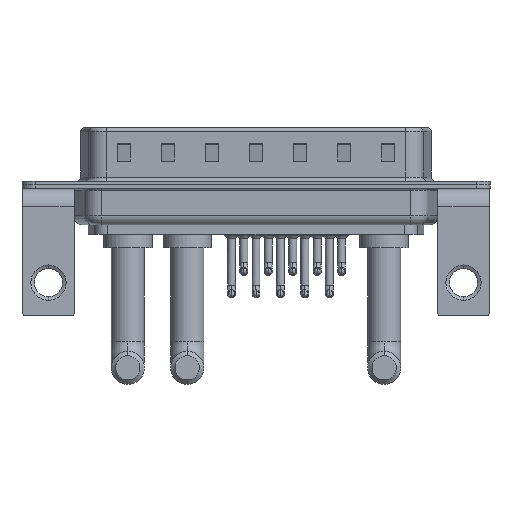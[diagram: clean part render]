
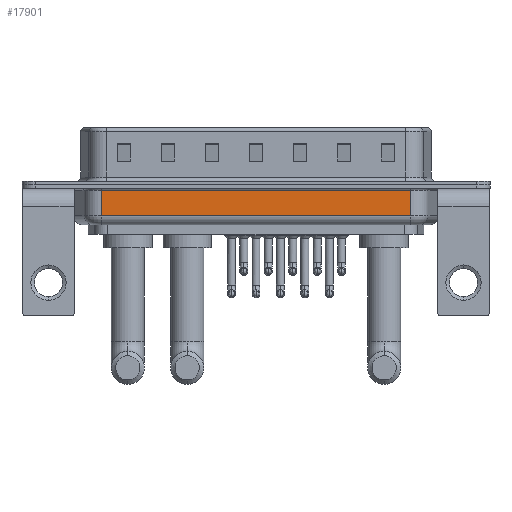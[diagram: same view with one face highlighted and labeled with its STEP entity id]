
A CAD part, front view. The second image highlights one B-rep face of the part: STEP entity #17901.
In plain terms, the highlighted planar face has unit normal (0, -1, 0).
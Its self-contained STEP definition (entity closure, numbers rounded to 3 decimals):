
#72 = VERTEX_POINT ( 'NONE', #9048 ) ;
#612 = CARTESIAN_POINT ( 'NONE',  ( 41.044, -5.35, -4.5 ) ) ;
#1063 = EDGE_CURVE ( 'NONE', #22351, #6361, #1485, .T. ) ;
#1106 = DIRECTION ( 'NONE',  ( 0., 0., 1. ) ) ;
#1122 = VECTOR ( 'NONE', #11524, 1000. ) ;
#1485 = LINE ( 'NONE', #7464, #18608 ) ;
#2270 = EDGE_CURVE ( 'NONE', #22351, #7087, #5910, .T. ) ;
#3722 = DIRECTION ( 'NONE',  ( 0., 0., 1. ) ) ;
#4683 = ORIENTED_EDGE ( 'NONE', *, *, #1063, .F. ) ;
#5135 = VECTOR ( 'NONE', #9587, 1000. ) ;
#5910 = LINE ( 'NONE', #15371, #7220 ) ;
#6139 = ORIENTED_EDGE ( 'NONE', *, *, #2270, .T. ) ;
#6293 = ORIENTED_EDGE ( 'NONE', *, *, #15575, .T. ) ;
#6361 = VERTEX_POINT ( 'NONE', #6918 ) ;
#6918 = CARTESIAN_POINT ( 'NONE',  ( 6.006, -5.35, -0.65 ) ) ;
#7087 = VERTEX_POINT ( 'NONE', #23111 ) ;
#7220 = VECTOR ( 'NONE', #13510, 1000. ) ;
#7464 = CARTESIAN_POINT ( 'NONE',  ( 6.006, -5.35, -4.5 ) ) ;
#9048 = CARTESIAN_POINT ( 'NONE',  ( 41.044, -5.35, -0.65 ) ) ;
#9587 = DIRECTION ( 'NONE',  ( 0., 0., 1. ) ) ;
#11524 = DIRECTION ( 'NONE',  ( -1., 0., 0. ) ) ;
#12431 = EDGE_LOOP ( 'NONE', ( #4683, #6139, #12727, #6293 ) ) ;
#12727 = ORIENTED_EDGE ( 'NONE', *, *, #16461, .T. ) ;
#13343 = LINE ( 'NONE', #612, #5135 ) ;
#13510 = DIRECTION ( 'NONE',  ( 1., 0., 0. ) ) ;
#14078 = CARTESIAN_POINT ( 'NONE',  ( 6.006, -5.35, -4.5 ) ) ;
#15163 = LINE ( 'NONE', #20838, #1122 ) ;
#15371 = CARTESIAN_POINT ( 'NONE',  ( 6.006, -5.35, -3.5 ) ) ;
#15575 = EDGE_CURVE ( 'NONE', #72, #6361, #15163, .T. ) ;
#15919 = PLANE ( 'NONE',  #16711 ) ;
#16461 = EDGE_CURVE ( 'NONE', #7087, #72, #13343, .T. ) ;
#16711 = AXIS2_PLACEMENT_3D ( 'NONE', #14078, #18139, #1106 ) ;
#17901 = ADVANCED_FACE ( 'NONE', ( #23459 ), #15919, .F. ) ;
#18139 = DIRECTION ( 'NONE',  ( 0., 1., 0. ) ) ;
#18608 = VECTOR ( 'NONE', #3722, 1000. ) ;
#18840 = CARTESIAN_POINT ( 'NONE',  ( 6.006, -5.35, -3.5 ) ) ;
#20838 = CARTESIAN_POINT ( 'NONE',  ( 6.006, -5.35, -0.65 ) ) ;
#22351 = VERTEX_POINT ( 'NONE', #18840 ) ;
#23111 = CARTESIAN_POINT ( 'NONE',  ( 41.044, -5.35, -3.5 ) ) ;
#23459 = FACE_OUTER_BOUND ( 'NONE', #12431, .T. ) ;
